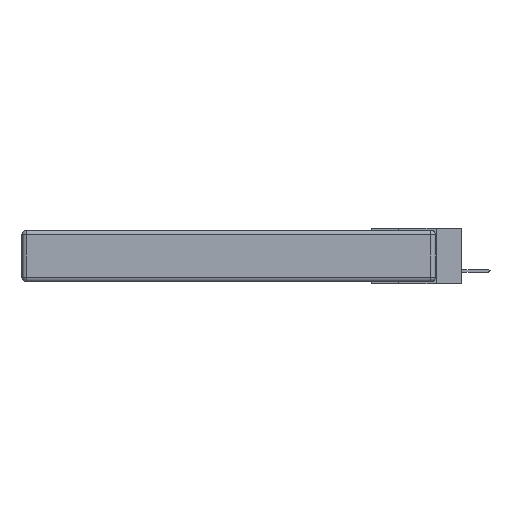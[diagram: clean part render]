
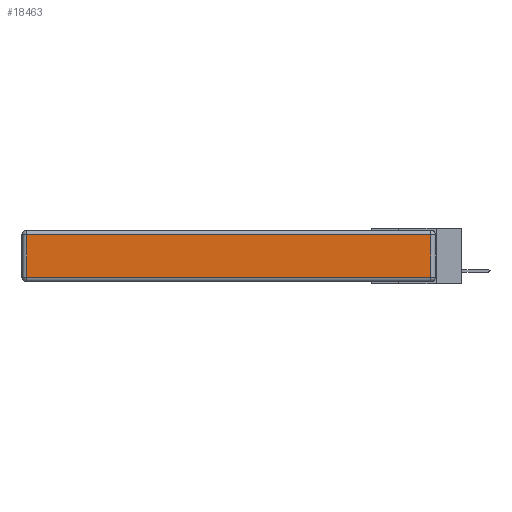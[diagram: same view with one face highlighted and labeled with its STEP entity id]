
A CAD part, left-side view. The second image highlights one B-rep face of the part: STEP entity #18463.
In plain terms, the highlighted planar face has unit normal (-1, 0, 0).
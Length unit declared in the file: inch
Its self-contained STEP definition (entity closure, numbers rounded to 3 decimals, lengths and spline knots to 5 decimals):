
#992 = LINE ( 'NONE', #4334, #11502 ) ;
#2132 = DIRECTION ( 'NONE',  ( 0., 0., 1. ) ) ;
#2568 = CARTESIAN_POINT ( 'NONE',  ( 0., 0., -0.343 ) ) ;
#4334 = CARTESIAN_POINT ( 'NONE',  ( 0., 2.75, -0.03 ) ) ;
#5235 = AXIS2_PLACEMENT_3D ( 'NONE', #2568, #30714, #2132 ) ;
#6758 = CARTESIAN_POINT ( 'NONE',  ( 0., 0.03, -0.313 ) ) ;
#7258 = EDGE_CURVE ( 'NONE', #16679, #25552, #22075, .T. ) ;
#8723 = VERTEX_POINT ( 'NONE', #9517 ) ;
#9072 = ORIENTED_EDGE ( 'NONE', *, *, #21776, .T. ) ;
#9517 = CARTESIAN_POINT ( 'NONE',  ( 0., 0.03, -0.03 ) ) ;
#9576 = DIRECTION ( 'NONE',  ( 0., 1., 0. ) ) ;
#10881 = CARTESIAN_POINT ( 'NONE',  ( 0., 0., -0.313 ) ) ;
#11502 = VECTOR ( 'NONE', #9576, 39.37008 ) ;
#12331 = PLANE ( 'NONE',  #5235 ) ;
#13512 = DIRECTION ( 'NONE',  ( 0., -1., 0. ) ) ;
#16679 = VERTEX_POINT ( 'NONE', #21826 ) ;
#17041 = VECTOR ( 'NONE', #18258, 39.37008 ) ;
#18112 = EDGE_CURVE ( 'NONE', #8723, #16679, #992, .T. ) ;
#18258 = DIRECTION ( 'NONE',  ( 0., 0., 1. ) ) ;
#18463 = ADVANCED_FACE ( 'NONE', ( #23311 ), #12331, .T. ) ;
#19874 = CARTESIAN_POINT ( 'NONE',  ( 0., 2.72, -0.313 ) ) ;
#21776 = EDGE_CURVE ( 'NONE', #26377, #8723, #23935, .T. ) ;
#21826 = CARTESIAN_POINT ( 'NONE',  ( 0., 2.72, -0.03 ) ) ;
#22075 = LINE ( 'NONE', #22219, #30594 ) ;
#22219 = CARTESIAN_POINT ( 'NONE',  ( 0., 2.72, -0.343 ) ) ;
#22473 = EDGE_CURVE ( 'NONE', #25552, #26377, #23445, .T. ) ;
#23311 = FACE_OUTER_BOUND ( 'NONE', #24173, .T. ) ;
#23445 = LINE ( 'NONE', #10881, #31124 ) ;
#23577 = CARTESIAN_POINT ( 'NONE',  ( 0., 0.03, -0.343 ) ) ;
#23935 = LINE ( 'NONE', #23577, #17041 ) ;
#24173 = EDGE_LOOP ( 'NONE', ( #33100, #9072, #26934, #27354 ) ) ;
#25552 = VERTEX_POINT ( 'NONE', #19874 ) ;
#26377 = VERTEX_POINT ( 'NONE', #6758 ) ;
#26934 = ORIENTED_EDGE ( 'NONE', *, *, #18112, .T. ) ;
#27354 = ORIENTED_EDGE ( 'NONE', *, *, #7258, .T. ) ;
#30594 = VECTOR ( 'NONE', #32848, 39.37008 ) ;
#30714 = DIRECTION ( 'NONE',  ( -1., 0., 0. ) ) ;
#31124 = VECTOR ( 'NONE', #13512, 39.37008 ) ;
#32848 = DIRECTION ( 'NONE',  ( 0., 0., -1. ) ) ;
#33100 = ORIENTED_EDGE ( 'NONE', *, *, #22473, .T. ) ;
